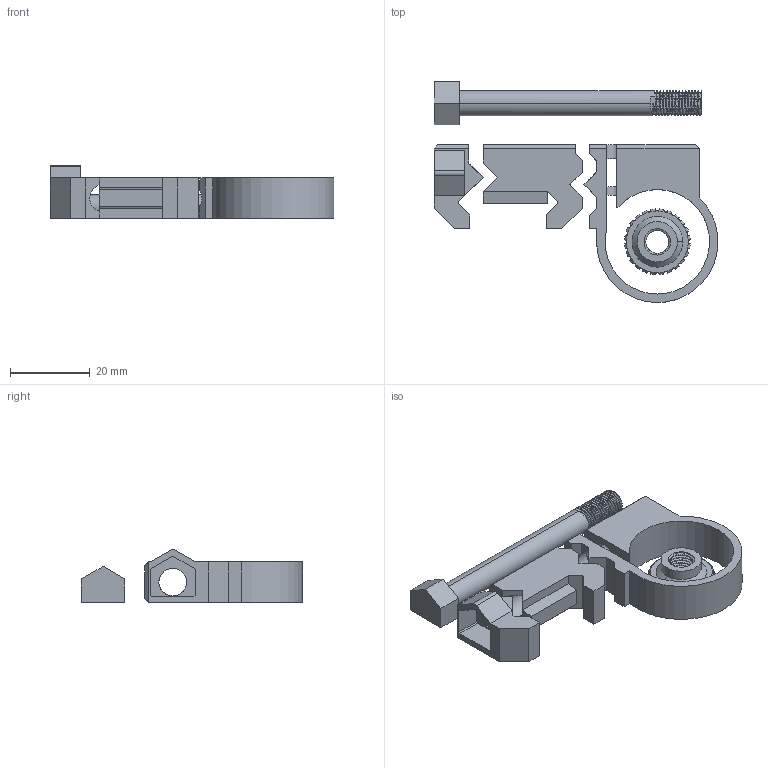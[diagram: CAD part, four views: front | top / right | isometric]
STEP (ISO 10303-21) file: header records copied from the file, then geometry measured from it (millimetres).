
FILE_DESCRIPTION (( 'STEP AP203' ), '1' );
FILE_NAME ('AF-WF-MI-MDL-001-STEP.STEP', '2020-07-21T23:53:35', ( '' ), ( '' ), 'SwSTEP 2.0', 'SolidWorks 2018', '' );
FILE_SCHEMA (( 'CONFIG_CONTROL_DESIGN' ));
Length unit declared in the file: inch
Products named in the file (1): AF-WF-MI-MDL-001-STEP
Bounding box: 71.25 x 55.48 x 13.24 mm (x, y, z)
Volume: 10804.2 mm3; surface area: 9705.8 mm2
Topology: 5 solids, 5 shells, 318 faces, 870 edges, 559 vertices
Faces by surface type: plane 131, cylinder 130, cone 50, bspline 7
Entity records: 15225 total; most frequent: CARTESIAN_POINT 7756, ORIENTED_EDGE 1740, DIRECTION 1320, EDGE_CURVE 870, VERTEX_POINT 559, AXIS2_PLACEMENT_3D 454, VECTOR 412, LINE 412
